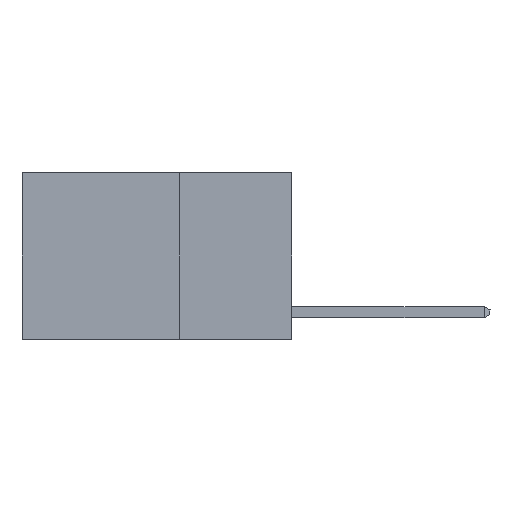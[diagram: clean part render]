
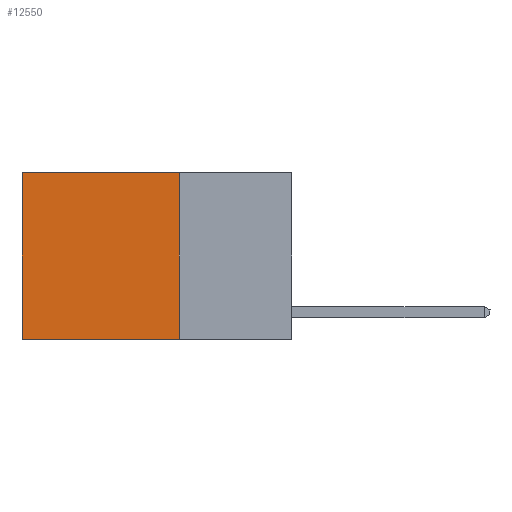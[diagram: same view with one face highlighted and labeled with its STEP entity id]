
A CAD part, left-side view. The second image highlights one B-rep face of the part: STEP entity #12550.
In plain terms, the highlighted planar face has unit normal (-1, 0, 0).
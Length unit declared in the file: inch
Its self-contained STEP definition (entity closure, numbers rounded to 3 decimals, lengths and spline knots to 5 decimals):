
#622 = EDGE_LOOP ( 'NONE', ( #6575, #9059, #11462, #2059 ) ) ;
#656 = LINE ( 'NONE', #8191, #13544 ) ;
#684 = VERTEX_POINT ( 'NONE', #12929 ) ;
#1109 = VERTEX_POINT ( 'NONE', #15796 ) ;
#1551 = EDGE_CURVE ( 'NONE', #1109, #684, #14244, .T. ) ;
#2059 = ORIENTED_EDGE ( 'NONE', *, *, #14404, .T. ) ;
#2129 = VERTEX_POINT ( 'NONE', #10533 ) ;
#4332 = VECTOR ( 'NONE', #5696, 39.37008 ) ;
#5034 = PLANE ( 'NONE',  #10552 ) ;
#5696 = DIRECTION ( 'NONE',  ( 0., 0., -1. ) ) ;
#5805 = LINE ( 'NONE', #12960, #12044 ) ;
#6198 = CARTESIAN_POINT ( 'NONE',  ( 0.2625, 0.25, -0.37 ) ) ;
#6325 = DIRECTION ( 'NONE',  ( 1., 0., 0. ) ) ;
#6575 = ORIENTED_EDGE ( 'NONE', *, *, #13704, .T. ) ;
#8191 = CARTESIAN_POINT ( 'NONE',  ( 0.2625, 0.25, 0. ) ) ;
#9059 = ORIENTED_EDGE ( 'NONE', *, *, #14670, .F. ) ;
#9079 = VERTEX_POINT ( 'NONE', #14242 ) ;
#9682 = LINE ( 'NONE', #6198, #10069 ) ;
#9752 = FACE_OUTER_BOUND ( 'NONE', #622, .T. ) ;
#10069 = VECTOR ( 'NONE', #13614, 39.37008 ) ;
#10533 = CARTESIAN_POINT ( 'NONE',  ( 0.2625, 0.6, -0.37 ) ) ;
#10552 = AXIS2_PLACEMENT_3D ( 'NONE', #12497, #6325, #14946 ) ;
#11462 = ORIENTED_EDGE ( 'NONE', *, *, #1551, .F. ) ;
#12044 = VECTOR ( 'NONE', #13012, 39.37008 ) ;
#12497 = CARTESIAN_POINT ( 'NONE',  ( 0.2625, 0.25, 0. ) ) ;
#12550 = ADVANCED_FACE ( 'NONE', ( #9752 ), #5034, .F. ) ;
#12929 = CARTESIAN_POINT ( 'NONE',  ( 0.2625, 0.25, -0.37 ) ) ;
#12960 = CARTESIAN_POINT ( 'NONE',  ( 0.2625, 0.6, 0. ) ) ;
#13012 = DIRECTION ( 'NONE',  ( 0., 0., -1. ) ) ;
#13142 = DIRECTION ( 'NONE',  ( 0., 1., 0. ) ) ;
#13544 = VECTOR ( 'NONE', #13142, 39.37008 ) ;
#13614 = DIRECTION ( 'NONE',  ( 0., 1., 0. ) ) ;
#13704 = EDGE_CURVE ( 'NONE', #9079, #2129, #5805, .T. ) ;
#14242 = CARTESIAN_POINT ( 'NONE',  ( 0.2625, 0.6, 0. ) ) ;
#14244 = LINE ( 'NONE', #14358, #4332 ) ;
#14358 = CARTESIAN_POINT ( 'NONE',  ( 0.2625, 0.25, 0. ) ) ;
#14404 = EDGE_CURVE ( 'NONE', #1109, #9079, #656, .T. ) ;
#14670 = EDGE_CURVE ( 'NONE', #684, #2129, #9682, .T. ) ;
#14946 = DIRECTION ( 'NONE',  ( 0., 0., -1. ) ) ;
#15796 = CARTESIAN_POINT ( 'NONE',  ( 0.2625, 0.25, 0. ) ) ;
